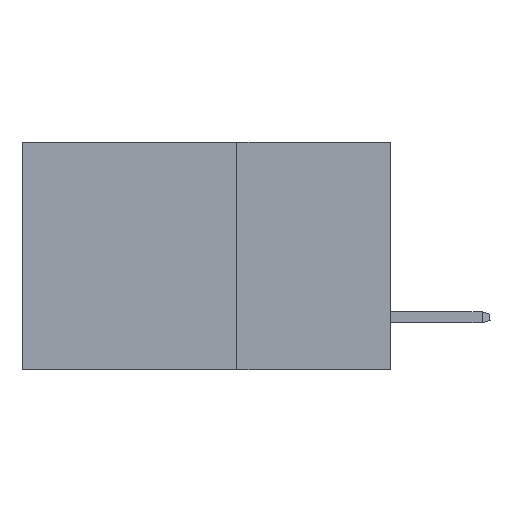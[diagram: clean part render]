
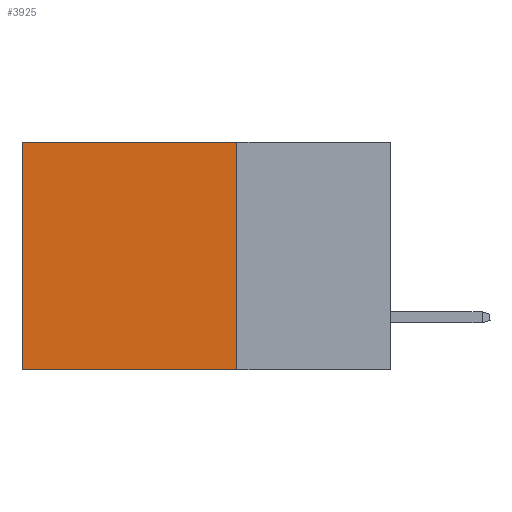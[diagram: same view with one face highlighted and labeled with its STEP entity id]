
A CAD part, left-side view. The second image highlights one B-rep face of the part: STEP entity #3925.
In plain terms, the highlighted planar face has unit normal (-1, 0, 0).
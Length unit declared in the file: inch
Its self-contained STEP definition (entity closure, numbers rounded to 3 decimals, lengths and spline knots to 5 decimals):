
#345 = VECTOR ( 'NONE', #7992, 39.37008 ) ;
#2222 = LINE ( 'NONE', #10525, #2937 ) ;
#2584 = VERTEX_POINT ( 'NONE', #13150 ) ;
#2864 = DIRECTION ( 'NONE',  ( 1., 0., 0. ) ) ;
#2937 = VECTOR ( 'NONE', #11704, 39.37008 ) ;
#2994 = EDGE_CURVE ( 'NONE', #6883, #8323, #10404, .T. ) ;
#3089 = VECTOR ( 'NONE', #9539, 39.37008 ) ;
#3925 = ADVANCED_FACE ( 'NONE', ( #12479 ), #9835, .F. ) ;
#4142 = VECTOR ( 'NONE', #10075, 39.37008 ) ;
#4143 = LINE ( 'NONE', #5438, #345 ) ;
#4316 = AXIS2_PLACEMENT_3D ( 'NONE', #12296, #2864, #5304 ) ;
#4689 = CARTESIAN_POINT ( 'NONE',  ( 0.2875, 0.6, 0. ) ) ;
#5304 = DIRECTION ( 'NONE',  ( 0., 0., -1. ) ) ;
#5438 = CARTESIAN_POINT ( 'NONE',  ( 0.2875, 0.25, 0. ) ) ;
#6168 = ORIENTED_EDGE ( 'NONE', *, *, #2994, .T. ) ;
#6222 = ORIENTED_EDGE ( 'NONE', *, *, #7148, .F. ) ;
#6676 = ORIENTED_EDGE ( 'NONE', *, *, #8851, .T. ) ;
#6883 = VERTEX_POINT ( 'NONE', #4689 ) ;
#7148 = EDGE_CURVE ( 'NONE', #12089, #8323, #2222, .T. ) ;
#7579 = LINE ( 'NONE', #14638, #4142 ) ;
#7992 = DIRECTION ( 'NONE',  ( 0., 0., -1. ) ) ;
#8323 = VERTEX_POINT ( 'NONE', #10975 ) ;
#8673 = CARTESIAN_POINT ( 'NONE',  ( 0.2875, 0.25, -0.37 ) ) ;
#8851 = EDGE_CURVE ( 'NONE', #2584, #6883, #7579, .T. ) ;
#9392 = EDGE_LOOP ( 'NONE', ( #6168, #6222, #11138, #6676 ) ) ;
#9539 = DIRECTION ( 'NONE',  ( 0., 0., -1. ) ) ;
#9835 = PLANE ( 'NONE',  #4316 ) ;
#10075 = DIRECTION ( 'NONE',  ( 0., 1., 0. ) ) ;
#10404 = LINE ( 'NONE', #10602, #3089 ) ;
#10525 = CARTESIAN_POINT ( 'NONE',  ( 0.2875, 0.25, -0.37 ) ) ;
#10602 = CARTESIAN_POINT ( 'NONE',  ( 0.2875, 0.6, 0. ) ) ;
#10975 = CARTESIAN_POINT ( 'NONE',  ( 0.2875, 0.6, -0.37 ) ) ;
#11138 = ORIENTED_EDGE ( 'NONE', *, *, #12130, .F. ) ;
#11704 = DIRECTION ( 'NONE',  ( 0., 1., 0. ) ) ;
#12089 = VERTEX_POINT ( 'NONE', #8673 ) ;
#12130 = EDGE_CURVE ( 'NONE', #2584, #12089, #4143, .T. ) ;
#12296 = CARTESIAN_POINT ( 'NONE',  ( 0.2875, 0.25, 0. ) ) ;
#12479 = FACE_OUTER_BOUND ( 'NONE', #9392, .T. ) ;
#13150 = CARTESIAN_POINT ( 'NONE',  ( 0.2875, 0.25, 0. ) ) ;
#14638 = CARTESIAN_POINT ( 'NONE',  ( 0.2875, 0.25, 0. ) ) ;
